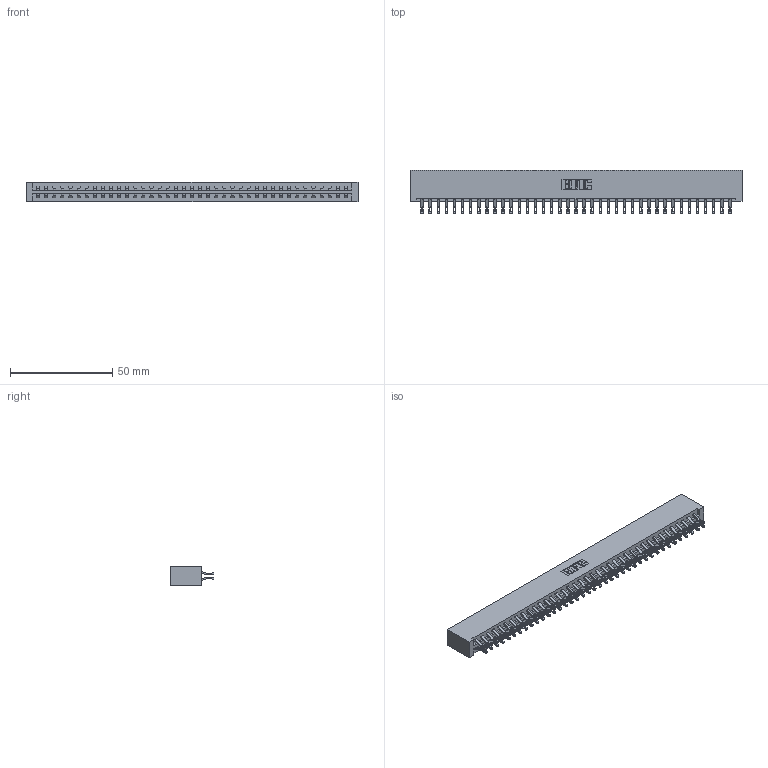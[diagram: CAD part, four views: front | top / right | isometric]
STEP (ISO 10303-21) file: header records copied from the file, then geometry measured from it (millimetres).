
FILE_DESCRIPTION (( 'STEP AP203' ), '1' );
FILE_NAME ('337-078-555-201.STEP', '2019-10-10T11:34:25', ( '' ), ( '' ), 'SwSTEP 2.0', 'SolidWorks 2016', '' );
FILE_SCHEMA (( 'CONFIG_CONTROL_DESIGN' ));
Length unit declared in the file: inch
Products named in the file (3): 337 Part_No Mounting Lugs; 337-078-555-201; 345-292-001_555 Tail
Assembly tree (79 placements, depth 2):
  337-078-555-201
    337 Part_No Mounting Lugs
    345-292-001_555 Tail  x78
Bounding box: 162.41 x 21.47 x 9.4 mm (x, y, z)
Volume: 18062.8 mm3; surface area: 21299.6 mm2
Topology: 79 solids, 79 shells, 4786 faces, 15029 edges, 10018 vertices
Faces by surface type: plane 2874, cylinder 1912
Entity records: 30675 total; most frequent: CARTESIAN_POINT 5204, ORIENTED_EDGE 5110, DIRECTION 4395, EDGE_CURVE 2555, LINE 2415, VECTOR 2415, VERTEX_POINT 1702, AXIS2_PLACEMENT_3D 990
